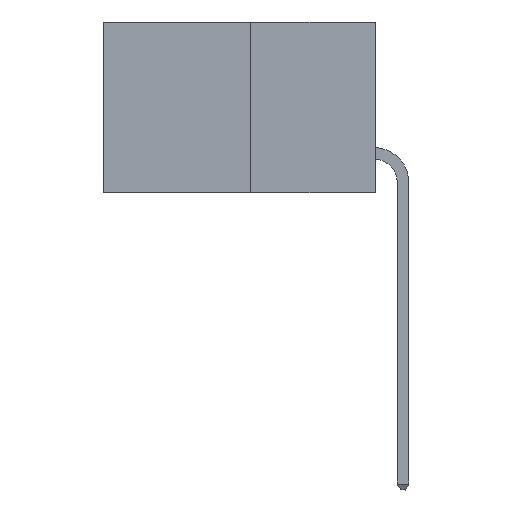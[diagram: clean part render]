
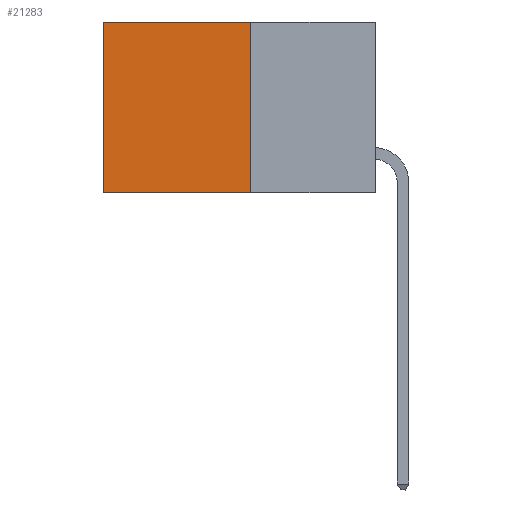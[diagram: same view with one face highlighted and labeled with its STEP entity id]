
A CAD part, left-side view. The second image highlights one B-rep face of the part: STEP entity #21283.
In plain terms, the highlighted planar face has unit normal (-1, 0, 0).
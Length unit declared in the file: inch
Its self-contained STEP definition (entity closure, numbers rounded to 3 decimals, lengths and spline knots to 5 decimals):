
#1551 = DIRECTION ( 'NONE',  ( 0., 1., 0. ) ) ;
#2228 = LINE ( 'NONE', #8278, #17212 ) ;
#2353 = EDGE_CURVE ( 'NONE', #19050, #19666, #2228, .T. ) ;
#2814 = CARTESIAN_POINT ( 'NONE',  ( 0.277, 0.59, -0.37 ) ) ;
#3356 = VERTEX_POINT ( 'NONE', #10702 ) ;
#3528 = CARTESIAN_POINT ( 'NONE',  ( 0.277, 0.27, -0.37 ) ) ;
#5577 = DIRECTION ( 'NONE',  ( 1., 0., 0. ) ) ;
#6082 = ORIENTED_EDGE ( 'NONE', *, *, #7279, .T. ) ;
#6116 = CARTESIAN_POINT ( 'NONE',  ( 0.277, 0.59, -0.37 ) ) ;
#6130 = LINE ( 'NONE', #15840, #16951 ) ;
#7279 = EDGE_CURVE ( 'NONE', #3356, #19118, #13897, .T. ) ;
#8278 = CARTESIAN_POINT ( 'NONE',  ( 0.277, 0.27, -0.37 ) ) ;
#8548 = CARTESIAN_POINT ( 'NONE',  ( 0.277, 0.27, 0. ) ) ;
#10702 = CARTESIAN_POINT ( 'NONE',  ( 0.277, 0.59, 0. ) ) ;
#12298 = EDGE_CURVE ( 'NONE', #19050, #3356, #13861, .T. ) ;
#12383 = ORIENTED_EDGE ( 'NONE', *, *, #2353, .F. ) ;
#13861 = LINE ( 'NONE', #8548, #24961 ) ;
#13897 = LINE ( 'NONE', #2814, #23869 ) ;
#15729 = PLANE ( 'NONE',  #20901 ) ;
#15840 = CARTESIAN_POINT ( 'NONE',  ( 0.277, 0.27, -0.37 ) ) ;
#16159 = CARTESIAN_POINT ( 'NONE',  ( 0.277, 0.27, -0.37 ) ) ;
#16722 = DIRECTION ( 'NONE',  ( 0., 1., 0. ) ) ;
#16951 = VECTOR ( 'NONE', #1551, 39.37008 ) ;
#17212 = VECTOR ( 'NONE', #18634, 39.37008 ) ;
#18113 = CARTESIAN_POINT ( 'NONE',  ( 0.277, 0.27, 0. ) ) ;
#18345 = EDGE_CURVE ( 'NONE', #19666, #19118, #6130, .T. ) ;
#18634 = DIRECTION ( 'NONE',  ( 0., 0., -1. ) ) ;
#18851 = ORIENTED_EDGE ( 'NONE', *, *, #12298, .T. ) ;
#19023 = ORIENTED_EDGE ( 'NONE', *, *, #18345, .F. ) ;
#19050 = VERTEX_POINT ( 'NONE', #18113 ) ;
#19118 = VERTEX_POINT ( 'NONE', #6116 ) ;
#19666 = VERTEX_POINT ( 'NONE', #16159 ) ;
#19772 = DIRECTION ( 'NONE',  ( 0., 0., -1. ) ) ;
#20511 = EDGE_LOOP ( 'NONE', ( #6082, #19023, #12383, #18851 ) ) ;
#20831 = FACE_OUTER_BOUND ( 'NONE', #20511, .T. ) ;
#20901 = AXIS2_PLACEMENT_3D ( 'NONE', #3528, #5577, #19772 ) ;
#21283 = ADVANCED_FACE ( 'NONE', ( #20831 ), #15729, .F. ) ;
#23289 = DIRECTION ( 'NONE',  ( 0., 0., -1. ) ) ;
#23869 = VECTOR ( 'NONE', #23289, 39.37008 ) ;
#24961 = VECTOR ( 'NONE', #16722, 39.37008 ) ;
